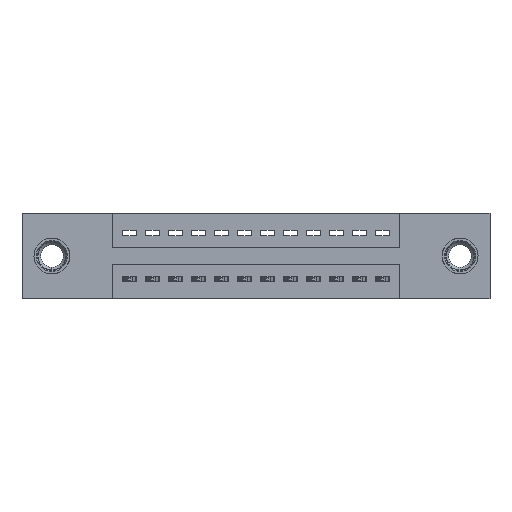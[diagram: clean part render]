
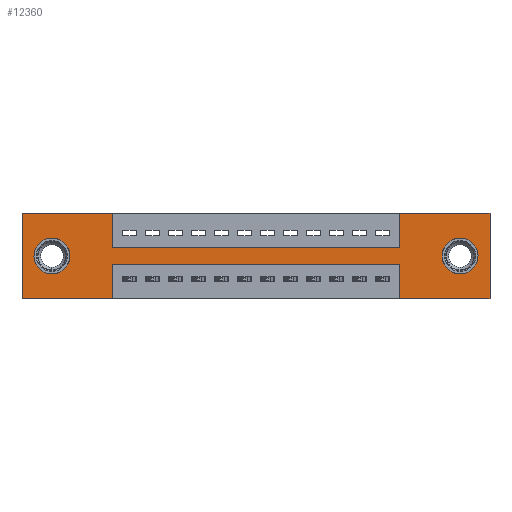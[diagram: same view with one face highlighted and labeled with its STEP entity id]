
A CAD part, front view. The second image highlights one B-rep face of the part: STEP entity #12360.
In plain terms, the highlighted planar face has unit normal (0, -1, 0).
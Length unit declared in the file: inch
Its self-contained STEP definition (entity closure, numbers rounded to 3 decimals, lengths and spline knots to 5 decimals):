
#50 = LINE ( 'NONE', #4450, #2769 ) ;
#125 = ORIENTED_EDGE ( 'NONE', *, *, #7967, .T. ) ;
#143 = EDGE_CURVE ( 'NONE', #6562, #2981, #7410, .T. ) ;
#184 = VERTEX_POINT ( 'NONE', #6653 ) ;
#306 = DIRECTION ( 'NONE',  ( 0., 0., -1. ) ) ;
#338 = ORIENTED_EDGE ( 'NONE', *, *, #628, .F. ) ;
#510 = ORIENTED_EDGE ( 'NONE', *, *, #14073, .F. ) ;
#569 = LINE ( 'NONE', #852, #11950 ) ;
#625 = VERTEX_POINT ( 'NONE', #2656 ) ;
#628 = EDGE_CURVE ( 'NONE', #13663, #6283, #3370, .T. ) ;
#849 = DIRECTION ( 'NONE',  ( 0., 0., -1. ) ) ;
#852 = CARTESIAN_POINT ( 'NONE',  ( 2.035, 0., 0. ) ) ;
#892 = ORIENTED_EDGE ( 'NONE', *, *, #2933, .F. ) ;
#1093 = CARTESIAN_POINT ( 'NONE',  ( 0., 0., 0. ) ) ;
#1096 = DIRECTION ( 'NONE',  ( 1., 0., 0. ) ) ;
#1139 = VERTEX_POINT ( 'NONE', #6188 ) ;
#1179 = VECTOR ( 'NONE', #12799, 39.37008 ) ;
#1338 = CARTESIAN_POINT ( 'NONE',  ( 0.3925, 0., -0.15 ) ) ;
#1507 = CARTESIAN_POINT ( 'NONE',  ( 1.6425, 0., -0.22 ) ) ;
#1529 = LINE ( 'NONE', #3390, #10024 ) ;
#1631 = VECTOR ( 'NONE', #1096, 39.37008 ) ;
#1632 = AXIS2_PLACEMENT_3D ( 'NONE', #5267, #2881, #10199 ) ;
#1673 = EDGE_CURVE ( 'NONE', #1139, #9565, #7193, .T. ) ;
#1969 = EDGE_CURVE ( 'NONE', #9565, #3292, #7828, .T. ) ;
#2094 = LINE ( 'NONE', #12443, #7694 ) ;
#2096 = DIRECTION ( 'NONE',  ( 1., 0., 0. ) ) ;
#2201 = DIRECTION ( 'NONE',  ( -1., 0., 0. ) ) ;
#2234 = AXIS2_PLACEMENT_3D ( 'NONE', #11960, #14145, #7713 ) ;
#2257 = CARTESIAN_POINT ( 'NONE',  ( 0.3925, 0., -0.22 ) ) ;
#2288 = CARTESIAN_POINT ( 'NONE',  ( 0., 0., 0. ) ) ;
#2656 = CARTESIAN_POINT ( 'NONE',  ( 1.6425, 0., -0.15 ) ) ;
#2736 = CARTESIAN_POINT ( 'NONE',  ( 0., 0., -0.37 ) ) ;
#2766 = CARTESIAN_POINT ( 'NONE',  ( 0.13, 0., -0.185 ) ) ;
#2769 = VECTOR ( 'NONE', #13150, 39.37008 ) ;
#2848 = FACE_BOUND ( 'NONE', #5107, .T. ) ;
#2881 = DIRECTION ( 'NONE',  ( 0., 1., 0. ) ) ;
#2933 = EDGE_CURVE ( 'NONE', #6283, #12923, #6774, .T. ) ;
#2981 = VERTEX_POINT ( 'NONE', #4778 ) ;
#3006 = CARTESIAN_POINT ( 'NONE',  ( 0.13, 0., -0.185 ) ) ;
#3115 = CARTESIAN_POINT ( 'NONE',  ( 2.035, 0., 0. ) ) ;
#3292 = VERTEX_POINT ( 'NONE', #2736 ) ;
#3370 = LINE ( 'NONE', #2288, #6034 ) ;
#3390 = CARTESIAN_POINT ( 'NONE',  ( 0.3925, 0., -0.15 ) ) ;
#3428 = AXIS2_PLACEMENT_3D ( 'NONE', #2766, #10444, #3877 ) ;
#3516 = EDGE_CURVE ( 'NONE', #13242, #6092, #5364, .T. ) ;
#3567 = EDGE_CURVE ( 'NONE', #6092, #11545, #569, .T. ) ;
#3787 = VECTOR ( 'NONE', #5089, 39.37008 ) ;
#3875 = ORIENTED_EDGE ( 'NONE', *, *, #1969, .F. ) ;
#3877 = DIRECTION ( 'NONE',  ( 0., 0., 1. ) ) ;
#3960 = EDGE_CURVE ( 'NONE', #5901, #1139, #9786, .T. ) ;
#4115 = DIRECTION ( 'NONE',  ( 0., 0., 1. ) ) ;
#4401 = VECTOR ( 'NONE', #5441, 39.37008 ) ;
#4431 = VERTEX_POINT ( 'NONE', #13363 ) ;
#4450 = CARTESIAN_POINT ( 'NONE',  ( 0., 0., 0. ) ) ;
#4515 = DIRECTION ( 'NONE',  ( 1., 0., 0. ) ) ;
#4518 = VECTOR ( 'NONE', #11196, 39.37008 ) ;
#4778 = CARTESIAN_POINT ( 'NONE',  ( 1.905, 0., -0.263 ) ) ;
#4909 = DIRECTION ( 'NONE',  ( 0., 0., 1. ) ) ;
#5089 = DIRECTION ( 'NONE',  ( 0., 0., -1. ) ) ;
#5107 = EDGE_LOOP ( 'NONE', ( #5427, #125 ) ) ;
#5267 = CARTESIAN_POINT ( 'NONE',  ( 1.905, 0., -0.185 ) ) ;
#5283 = CARTESIAN_POINT ( 'NONE',  ( 0.3925, 0., 0. ) ) ;
#5364 = LINE ( 'NONE', #1093, #1631 ) ;
#5427 = ORIENTED_EDGE ( 'NONE', *, *, #8079, .T. ) ;
#5441 = DIRECTION ( 'NONE',  ( -1., 0., 0. ) ) ;
#5563 = EDGE_CURVE ( 'NONE', #11545, #4431, #12752, .T. ) ;
#5673 = EDGE_LOOP ( 'NONE', ( #11732, #13027, #6271, #14275, #12371, #12467, #12452, #10862, #892, #338, #510, #3875 ) ) ;
#5901 = VERTEX_POINT ( 'NONE', #1507 ) ;
#6034 = VECTOR ( 'NONE', #2096, 39.37008 ) ;
#6053 = VECTOR ( 'NONE', #8942, 39.37008 ) ;
#6092 = VERTEX_POINT ( 'NONE', #3115 ) ;
#6188 = CARTESIAN_POINT ( 'NONE',  ( 0.3925, 0., -0.22 ) ) ;
#6271 = ORIENTED_EDGE ( 'NONE', *, *, #6970, .F. ) ;
#6283 = VERTEX_POINT ( 'NONE', #6834 ) ;
#6562 = VERTEX_POINT ( 'NONE', #7495 ) ;
#6576 = CARTESIAN_POINT ( 'NONE',  ( 0., 0., -0.37 ) ) ;
#6627 = PLANE ( 'NONE',  #2234 ) ;
#6653 = CARTESIAN_POINT ( 'NONE',  ( 0.13, 0., -0.107 ) ) ;
#6774 = LINE ( 'NONE', #5283, #3787 ) ;
#6834 = CARTESIAN_POINT ( 'NONE',  ( 0.3925, 0., 0. ) ) ;
#6970 = EDGE_CURVE ( 'NONE', #4431, #5901, #2094, .T. ) ;
#7077 = DIRECTION ( 'NONE',  ( 0., 1., 0. ) ) ;
#7193 = LINE ( 'NONE', #12818, #1179 ) ;
#7410 = CIRCLE ( 'NONE', #1632, 0.078 ) ;
#7495 = CARTESIAN_POINT ( 'NONE',  ( 1.905, 0., -0.107 ) ) ;
#7694 = VECTOR ( 'NONE', #4909, 39.37008 ) ;
#7713 = DIRECTION ( 'NONE',  ( 0., 0., -1. ) ) ;
#7828 = LINE ( 'NONE', #11262, #4518 ) ;
#7967 = EDGE_CURVE ( 'NONE', #14081, #184, #10007, .T. ) ;
#8079 = EDGE_CURVE ( 'NONE', #184, #14081, #14048, .T. ) ;
#8460 = CARTESIAN_POINT ( 'NONE',  ( 2.035, 0., -0.37 ) ) ;
#8585 = AXIS2_PLACEMENT_3D ( 'NONE', #13513, #7077, #306 ) ;
#8742 = FACE_OUTER_BOUND ( 'NONE', #5673, .T. ) ;
#8942 = DIRECTION ( 'NONE',  ( 0., 0., 1. ) ) ;
#9280 = LINE ( 'NONE', #12104, #6053 ) ;
#9565 = VERTEX_POINT ( 'NONE', #11001 ) ;
#9786 = LINE ( 'NONE', #2257, #12630 ) ;
#10007 = CIRCLE ( 'NONE', #3428, 0.078 ) ;
#10024 = VECTOR ( 'NONE', #4515, 39.37008 ) ;
#10199 = DIRECTION ( 'NONE',  ( 0., 0., -1. ) ) ;
#10349 = CARTESIAN_POINT ( 'NONE',  ( 0., 0., 0. ) ) ;
#10444 = DIRECTION ( 'NONE',  ( 0., 1., 0. ) ) ;
#10569 = EDGE_CURVE ( 'NONE', #625, #13242, #9280, .T. ) ;
#10673 = DIRECTION ( 'NONE',  ( 0., 1., 0. ) ) ;
#10862 = ORIENTED_EDGE ( 'NONE', *, *, #13451, .F. ) ;
#11001 = CARTESIAN_POINT ( 'NONE',  ( 0.3925, 0., -0.37 ) ) ;
#11196 = DIRECTION ( 'NONE',  ( -1., 0., 0. ) ) ;
#11235 = FACE_BOUND ( 'NONE', #12244, .T. ) ;
#11262 = CARTESIAN_POINT ( 'NONE',  ( 0., 0., -0.37 ) ) ;
#11343 = EDGE_CURVE ( 'NONE', #2981, #6562, #12945, .T. ) ;
#11496 = AXIS2_PLACEMENT_3D ( 'NONE', #3006, #10673, #4115 ) ;
#11545 = VERTEX_POINT ( 'NONE', #8460 ) ;
#11732 = ORIENTED_EDGE ( 'NONE', *, *, #1673, .F. ) ;
#11950 = VECTOR ( 'NONE', #849, 39.37008 ) ;
#11960 = CARTESIAN_POINT ( 'NONE',  ( 0., 0., -0.37 ) ) ;
#12104 = CARTESIAN_POINT ( 'NONE',  ( 1.6425, 0., 0. ) ) ;
#12244 = EDGE_LOOP ( 'NONE', ( #13170, #12773 ) ) ;
#12360 = ADVANCED_FACE ( 'NONE', ( #11235, #2848, #8742 ), #6627, .T. ) ;
#12371 = ORIENTED_EDGE ( 'NONE', *, *, #3567, .F. ) ;
#12443 = CARTESIAN_POINT ( 'NONE',  ( 1.6425, 0., -0.37 ) ) ;
#12452 = ORIENTED_EDGE ( 'NONE', *, *, #10569, .F. ) ;
#12467 = ORIENTED_EDGE ( 'NONE', *, *, #3516, .F. ) ;
#12630 = VECTOR ( 'NONE', #2201, 39.37008 ) ;
#12752 = LINE ( 'NONE', #6576, #4401 ) ;
#12773 = ORIENTED_EDGE ( 'NONE', *, *, #11343, .T. ) ;
#12799 = DIRECTION ( 'NONE',  ( 0., 0., -1. ) ) ;
#12818 = CARTESIAN_POINT ( 'NONE',  ( 0.3925, 0., -0.37 ) ) ;
#12923 = VERTEX_POINT ( 'NONE', #1338 ) ;
#12945 = CIRCLE ( 'NONE', #8585, 0.078 ) ;
#13027 = ORIENTED_EDGE ( 'NONE', *, *, #3960, .F. ) ;
#13150 = DIRECTION ( 'NONE',  ( 0., 0., 1. ) ) ;
#13170 = ORIENTED_EDGE ( 'NONE', *, *, #143, .T. ) ;
#13242 = VERTEX_POINT ( 'NONE', #13884 ) ;
#13363 = CARTESIAN_POINT ( 'NONE',  ( 1.6425, 0., -0.37 ) ) ;
#13451 = EDGE_CURVE ( 'NONE', #12923, #625, #1529, .T. ) ;
#13513 = CARTESIAN_POINT ( 'NONE',  ( 1.905, 0., -0.185 ) ) ;
#13663 = VERTEX_POINT ( 'NONE', #10349 ) ;
#13884 = CARTESIAN_POINT ( 'NONE',  ( 1.6425, 0., 0. ) ) ;
#14048 = CIRCLE ( 'NONE', #11496, 0.078 ) ;
#14073 = EDGE_CURVE ( 'NONE', #3292, #13663, #50, .T. ) ;
#14081 = VERTEX_POINT ( 'NONE', #14230 ) ;
#14145 = DIRECTION ( 'NONE',  ( 0., -1., 0. ) ) ;
#14230 = CARTESIAN_POINT ( 'NONE',  ( 0.13, 0., -0.263 ) ) ;
#14275 = ORIENTED_EDGE ( 'NONE', *, *, #5563, .F. ) ;
